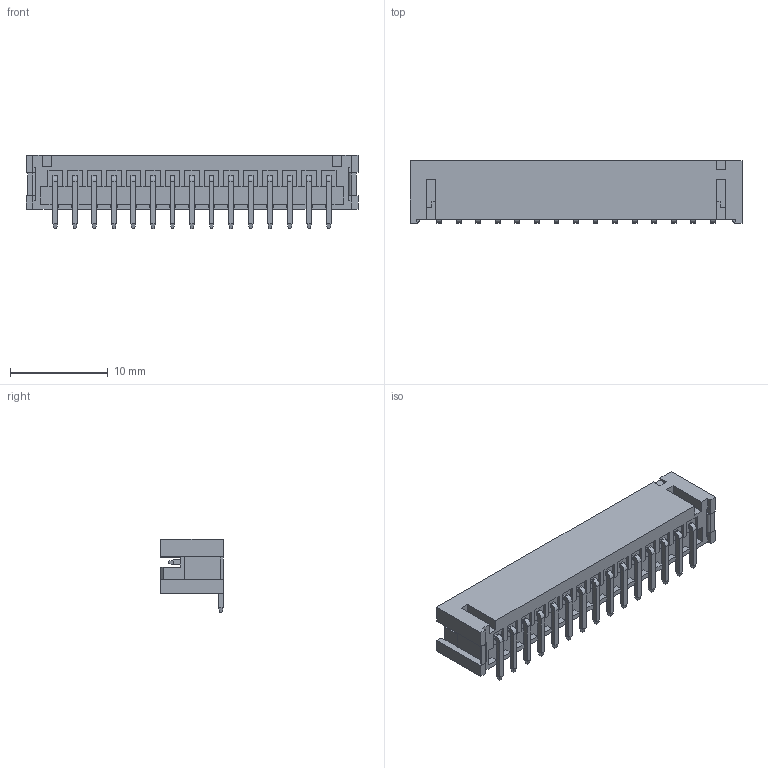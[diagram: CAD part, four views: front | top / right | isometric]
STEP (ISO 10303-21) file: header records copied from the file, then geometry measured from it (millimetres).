
FILE_DESCRIPTION (( 'STEP AP203' ), '1' );
FILE_NAME ('140-515-417-011.STEP', '2020-03-31T20:08:04', ( '' ), ( '' ), 'SwSTEP 2.0', 'SolidWorks 2016', '' );
FILE_SCHEMA (( 'CONFIG_CONTROL_DESIGN' ));
Length unit declared in the file: millimetre
Products named in the file (4): V SMT Pad; V SMT Contact; 140-515-417-011; V SMT Housing_515
Assembly tree (18 placements, depth 2):
  140-515-417-011
    V SMT Housing_515
    V SMT Contact  x15
    V SMT Pad  x2
Bounding box: 34 x 6.4 x 7.5 mm (x, y, z)
Volume: 480.3 mm3; surface area: 1743.1 mm2
Topology: 18 solids, 18 shells, 670 faces, 1664 edges, 1026 vertices
Faces by surface type: plane 636, cylinder 34
Entity records: 12178 total; most frequent: CARTESIAN_POINT 2047, ORIENTED_EDGE 2024, DIRECTION 1758, EDGE_CURVE 1012, VECTOR 1004, LINE 1004, VERTEX_POINT 666, EDGE_LOOP 378
